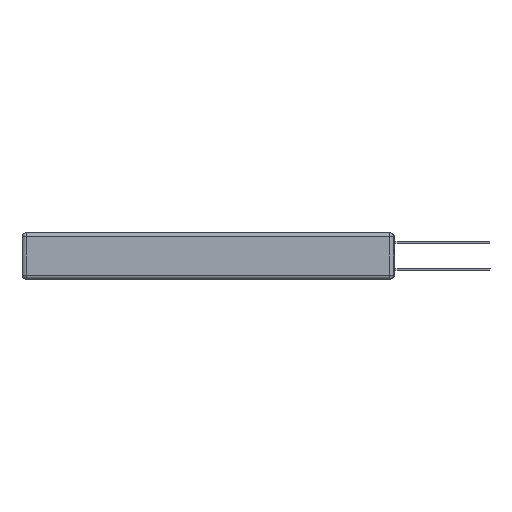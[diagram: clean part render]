
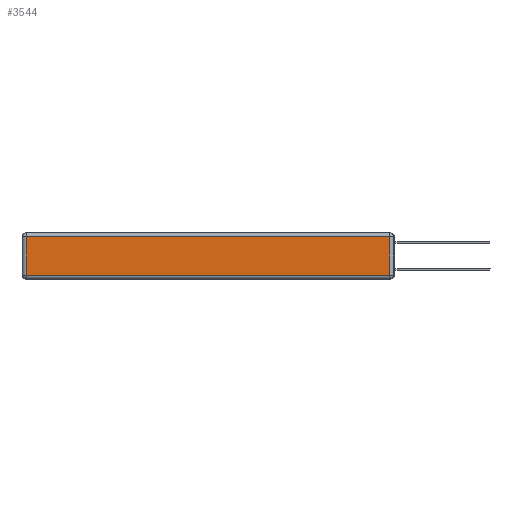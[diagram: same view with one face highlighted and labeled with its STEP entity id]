
A CAD part, left-side view. The second image highlights one B-rep face of the part: STEP entity #3544.
In plain terms, the highlighted planar face has unit normal (-1, 0, 0).
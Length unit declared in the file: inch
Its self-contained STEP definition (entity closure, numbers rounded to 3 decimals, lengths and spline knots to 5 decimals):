
#7 = VERTEX_POINT ( 'NONE', #16027 ) ;
#140 = CARTESIAN_POINT ( 'NONE',  ( 0., 2.72, -0.343 ) ) ;
#590 = VECTOR ( 'NONE', #1413, 39.37008 ) ;
#806 = VERTEX_POINT ( 'NONE', #9768 ) ;
#1413 = DIRECTION ( 'NONE',  ( 0., 0., -1. ) ) ;
#2103 = LINE ( 'NONE', #4845, #10278 ) ;
#2418 = EDGE_CURVE ( 'NONE', #806, #12098, #13819, .T. ) ;
#3110 = DIRECTION ( 'NONE',  ( 0., -1., 0. ) ) ;
#3544 = ADVANCED_FACE ( 'NONE', ( #4199 ), #5499, .T. ) ;
#4199 = FACE_OUTER_BOUND ( 'NONE', #11437, .T. ) ;
#4335 = ORIENTED_EDGE ( 'NONE', *, *, #2418, .T. ) ;
#4845 = CARTESIAN_POINT ( 'NONE',  ( 0., 0.03, -0.343 ) ) ;
#5499 = PLANE ( 'NONE',  #6916 ) ;
#5755 = DIRECTION ( 'NONE',  ( -1., 0., 0. ) ) ;
#6134 = EDGE_CURVE ( 'NONE', #7, #806, #17519, .T. ) ;
#6916 = AXIS2_PLACEMENT_3D ( 'NONE', #9729, #5755, #12347 ) ;
#7859 = DIRECTION ( 'NONE',  ( 0., 1., 0. ) ) ;
#7938 = VECTOR ( 'NONE', #3110, 39.37008 ) ;
#8746 = CARTESIAN_POINT ( 'NONE',  ( 0., 0., -0.313 ) ) ;
#9209 = CARTESIAN_POINT ( 'NONE',  ( 0., 2.75, -0.03 ) ) ;
#9458 = ORIENTED_EDGE ( 'NONE', *, *, #10134, .T. ) ;
#9729 = CARTESIAN_POINT ( 'NONE',  ( 0., 0., -0.343 ) ) ;
#9768 = CARTESIAN_POINT ( 'NONE',  ( 0., 2.72, -0.03 ) ) ;
#10134 = EDGE_CURVE ( 'NONE', #12098, #12409, #16583, .T. ) ;
#10278 = VECTOR ( 'NONE', #13071, 39.37008 ) ;
#11072 = ORIENTED_EDGE ( 'NONE', *, *, #11624, .T. ) ;
#11437 = EDGE_LOOP ( 'NONE', ( #9458, #11072, #16925, #4335 ) ) ;
#11624 = EDGE_CURVE ( 'NONE', #12409, #7, #2103, .T. ) ;
#12098 = VERTEX_POINT ( 'NONE', #13738 ) ;
#12347 = DIRECTION ( 'NONE',  ( 0., 0., 1. ) ) ;
#12409 = VERTEX_POINT ( 'NONE', #15979 ) ;
#13071 = DIRECTION ( 'NONE',  ( 0., 0., 1. ) ) ;
#13738 = CARTESIAN_POINT ( 'NONE',  ( 0., 2.72, -0.313 ) ) ;
#13819 = LINE ( 'NONE', #140, #590 ) ;
#15979 = CARTESIAN_POINT ( 'NONE',  ( 0., 0.03, -0.313 ) ) ;
#16027 = CARTESIAN_POINT ( 'NONE',  ( 0., 0.03, -0.03 ) ) ;
#16583 = LINE ( 'NONE', #8746, #7938 ) ;
#16789 = VECTOR ( 'NONE', #7859, 39.37008 ) ;
#16925 = ORIENTED_EDGE ( 'NONE', *, *, #6134, .T. ) ;
#17519 = LINE ( 'NONE', #9209, #16789 ) ;
